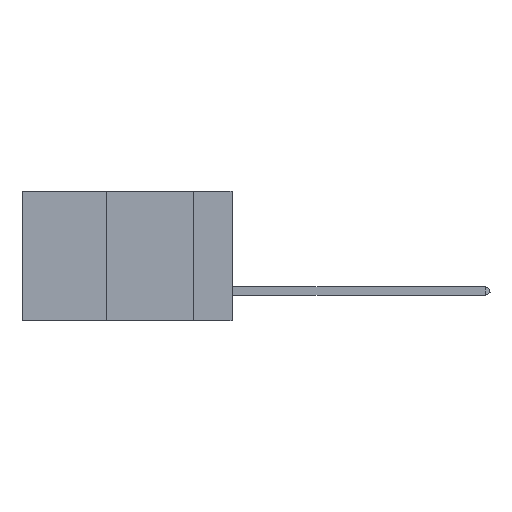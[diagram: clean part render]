
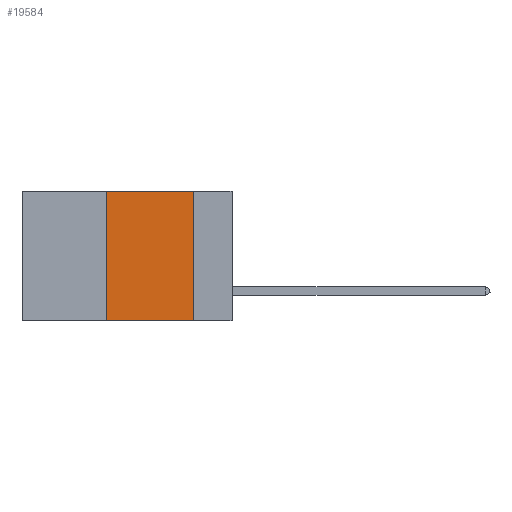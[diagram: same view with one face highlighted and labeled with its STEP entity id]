
A CAD part, left-side view. The second image highlights one B-rep face of the part: STEP entity #19584.
In plain terms, the highlighted planar face has unit normal (-1, 0, 0).
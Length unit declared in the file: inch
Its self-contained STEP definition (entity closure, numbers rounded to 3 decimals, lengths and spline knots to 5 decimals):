
#562 = CARTESIAN_POINT ( 'NONE',  ( 0., 0.6, 0. ) ) ;
#921 = CARTESIAN_POINT ( 'NONE',  ( 0., 0.11, 0. ) ) ;
#1250 = VERTEX_POINT ( 'NONE', #921 ) ;
#1374 = CARTESIAN_POINT ( 'NONE',  ( 0., 0.11, 0. ) ) ;
#1861 = CARTESIAN_POINT ( 'NONE',  ( 0., 0.36, 0. ) ) ;
#1975 = CARTESIAN_POINT ( 'NONE',  ( 0., 0.6, -0.37 ) ) ;
#2175 = DIRECTION ( 'NONE',  ( 0., 0., -1. ) ) ;
#3069 = LINE ( 'NONE', #562, #14369 ) ;
#3968 = ORIENTED_EDGE ( 'NONE', *, *, #10832, .F. ) ;
#4044 = DIRECTION ( 'NONE',  ( 0., -1., 0. ) ) ;
#4475 = VECTOR ( 'NONE', #15758, 39.37008 ) ;
#4705 = EDGE_CURVE ( 'NONE', #14663, #13197, #9610, .T. ) ;
#5812 = DIRECTION ( 'NONE',  ( 0., 0., -1. ) ) ;
#7022 = VERTEX_POINT ( 'NONE', #17774 ) ;
#8575 = EDGE_CURVE ( 'NONE', #13197, #1250, #3069, .T. ) ;
#8767 = CARTESIAN_POINT ( 'NONE',  ( 0., 0.36, 0. ) ) ;
#9610 = LINE ( 'NONE', #8767, #17326 ) ;
#10158 = CARTESIAN_POINT ( 'NONE',  ( 0., 0.6, 0. ) ) ;
#10705 = FACE_OUTER_BOUND ( 'NONE', #13810, .T. ) ;
#10832 = EDGE_CURVE ( 'NONE', #1250, #7022, #11676, .T. ) ;
#10860 = EDGE_CURVE ( 'NONE', #14663, #7022, #16006, .T. ) ;
#11676 = LINE ( 'NONE', #1374, #14058 ) ;
#11706 = DIRECTION ( 'NONE',  ( 1., 0., 0. ) ) ;
#13197 = VERTEX_POINT ( 'NONE', #1861 ) ;
#13449 = PLANE ( 'NONE',  #19071 ) ;
#13810 = EDGE_LOOP ( 'NONE', ( #3968, #17924, #15460, #18124 ) ) ;
#14058 = VECTOR ( 'NONE', #2175, 39.37008 ) ;
#14369 = VECTOR ( 'NONE', #4044, 39.37008 ) ;
#14663 = VERTEX_POINT ( 'NONE', #14974 ) ;
#14974 = CARTESIAN_POINT ( 'NONE',  ( 0., 0.36, -0.37 ) ) ;
#15460 = ORIENTED_EDGE ( 'NONE', *, *, #4705, .F. ) ;
#15758 = DIRECTION ( 'NONE',  ( 0., -1., 0. ) ) ;
#16006 = LINE ( 'NONE', #1975, #4475 ) ;
#17326 = VECTOR ( 'NONE', #18237, 39.37008 ) ;
#17774 = CARTESIAN_POINT ( 'NONE',  ( 0., 0.11, -0.37 ) ) ;
#17924 = ORIENTED_EDGE ( 'NONE', *, *, #8575, .F. ) ;
#18124 = ORIENTED_EDGE ( 'NONE', *, *, #10860, .T. ) ;
#18237 = DIRECTION ( 'NONE',  ( 0., 0., 1. ) ) ;
#19071 = AXIS2_PLACEMENT_3D ( 'NONE', #10158, #11706, #5812 ) ;
#19584 = ADVANCED_FACE ( 'NONE', ( #10705 ), #13449, .F. ) ;
